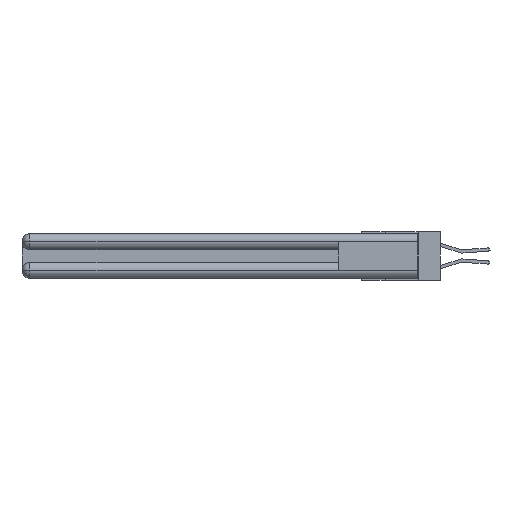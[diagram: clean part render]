
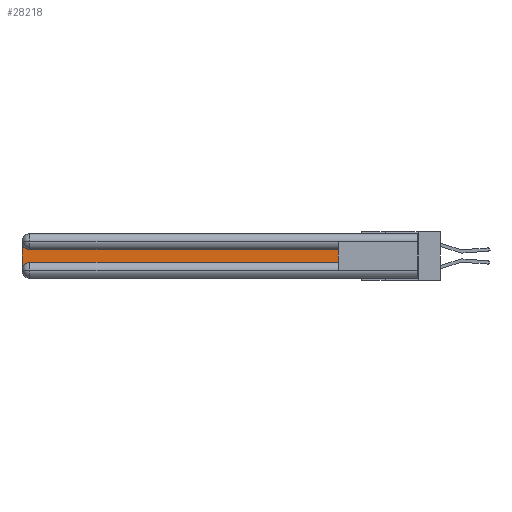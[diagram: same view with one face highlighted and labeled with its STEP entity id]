
A CAD part, left-side view. The second image highlights one B-rep face of the part: STEP entity #28218.
In plain terms, the highlighted planar face has unit normal (-1, 0, 0).
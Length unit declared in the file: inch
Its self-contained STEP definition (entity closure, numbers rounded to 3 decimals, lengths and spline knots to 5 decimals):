
#247 = LINE ( 'NONE', #579, #2518 ) ;
#422 = VERTEX_POINT ( 'NONE', #16018 ) ;
#579 = CARTESIAN_POINT ( 'NONE',  ( 0.075, 0.6, -0.2175 ) ) ;
#865 = CIRCLE ( 'NONE', #6134, 0.06 ) ;
#1086 = VERTEX_POINT ( 'NONE', #16862 ) ;
#1247 = VERTEX_POINT ( 'NONE', #30723 ) ;
#1256 = CARTESIAN_POINT ( 'NONE',  ( 0.075, 0.6, -0.1225 ) ) ;
#1810 = VECTOR ( 'NONE', #14189, 39.37008 ) ;
#2518 = VECTOR ( 'NONE', #12991, 39.37008 ) ;
#2558 = VERTEX_POINT ( 'NONE', #23196 ) ;
#3479 = VECTOR ( 'NONE', #5385, 39.37008 ) ;
#3515 = ORIENTED_EDGE ( 'NONE', *, *, #16739, .T. ) ;
#3923 = PLANE ( 'NONE',  #14638 ) ;
#5242 = CARTESIAN_POINT ( 'NONE',  ( 0.075, 3., -0.2175 ) ) ;
#5385 = DIRECTION ( 'NONE',  ( 0., 0., -1. ) ) ;
#5862 = CARTESIAN_POINT ( 'NONE',  ( 0.075, 2.94, -0.2175 ) ) ;
#6134 = AXIS2_PLACEMENT_3D ( 'NONE', #11601, #14155, #9061 ) ;
#6903 = DIRECTION ( 'NONE',  ( 0., 0., 1. ) ) ;
#7450 = CARTESIAN_POINT ( 'NONE',  ( 0.075, 3., -0.2775 ) ) ;
#7666 = CARTESIAN_POINT ( 'NONE',  ( 0.075, 2.94, -0.2775 ) ) ;
#8830 = DIRECTION ( 'NONE',  ( 1., 0., 0. ) ) ;
#9061 = DIRECTION ( 'NONE',  ( 0., 0., -1. ) ) ;
#9921 = ORIENTED_EDGE ( 'NONE', *, *, #21133, .T. ) ;
#10585 = EDGE_CURVE ( 'NONE', #2558, #15244, #20259, .T. ) ;
#11601 = CARTESIAN_POINT ( 'NONE',  ( 0.075, 2.94, -0.0625 ) ) ;
#12400 = ORIENTED_EDGE ( 'NONE', *, *, #17085, .T. ) ;
#12991 = DIRECTION ( 'NONE',  ( 0., -1., 0. ) ) ;
#14155 = DIRECTION ( 'NONE',  ( 1., 0., 0. ) ) ;
#14189 = DIRECTION ( 'NONE',  ( 0., 1., 0. ) ) ;
#14638 = AXIS2_PLACEMENT_3D ( 'NONE', #25776, #8830, #30694 ) ;
#15244 = VERTEX_POINT ( 'NONE', #7450 ) ;
#15959 = ORIENTED_EDGE ( 'NONE', *, *, #24954, .T. ) ;
#16018 = CARTESIAN_POINT ( 'NONE',  ( 0.075, 0.6, -0.2175 ) ) ;
#16739 = EDGE_CURVE ( 'NONE', #21517, #422, #247, .T. ) ;
#16862 = CARTESIAN_POINT ( 'NONE',  ( 0.075, 2.94, -0.1225 ) ) ;
#17085 = EDGE_CURVE ( 'NONE', #422, #1247, #24222, .T. ) ;
#17990 = CIRCLE ( 'NONE', #30659, 0.06 ) ;
#19345 = CARTESIAN_POINT ( 'NONE',  ( 0.075, 0.6, -0.2175 ) ) ;
#20259 = LINE ( 'NONE', #5242, #3479 ) ;
#21133 = EDGE_CURVE ( 'NONE', #15244, #21517, #17990, .T. ) ;
#21162 = VECTOR ( 'NONE', #6903, 39.37008 ) ;
#21517 = VERTEX_POINT ( 'NONE', #5862 ) ;
#21734 = EDGE_CURVE ( 'NONE', #1086, #2558, #865, .T. ) ;
#23196 = CARTESIAN_POINT ( 'NONE',  ( 0.075, 3., -0.0625 ) ) ;
#24222 = LINE ( 'NONE', #19345, #21162 ) ;
#24954 = EDGE_CURVE ( 'NONE', #1247, #1086, #25774, .T. ) ;
#25774 = LINE ( 'NONE', #1256, #1810 ) ;
#25776 = CARTESIAN_POINT ( 'NONE',  ( 0.075, 3., -0.1225 ) ) ;
#26968 = DIRECTION ( 'NONE',  ( 0., 0., -1. ) ) ;
#27172 = DIRECTION ( 'NONE',  ( 1., 0., 0. ) ) ;
#28218 = ADVANCED_FACE ( 'NONE', ( #29502 ), #3923, .F. ) ;
#29136 = ORIENTED_EDGE ( 'NONE', *, *, #10585, .T. ) ;
#29403 = ORIENTED_EDGE ( 'NONE', *, *, #21734, .T. ) ;
#29502 = FACE_OUTER_BOUND ( 'NONE', #30525, .T. ) ;
#30525 = EDGE_LOOP ( 'NONE', ( #15959, #29403, #29136, #9921, #3515, #12400 ) ) ;
#30659 = AXIS2_PLACEMENT_3D ( 'NONE', #7666, #27172, #26968 ) ;
#30694 = DIRECTION ( 'NONE',  ( 0., 0., -1. ) ) ;
#30723 = CARTESIAN_POINT ( 'NONE',  ( 0.075, 0.6, -0.1225 ) ) ;
